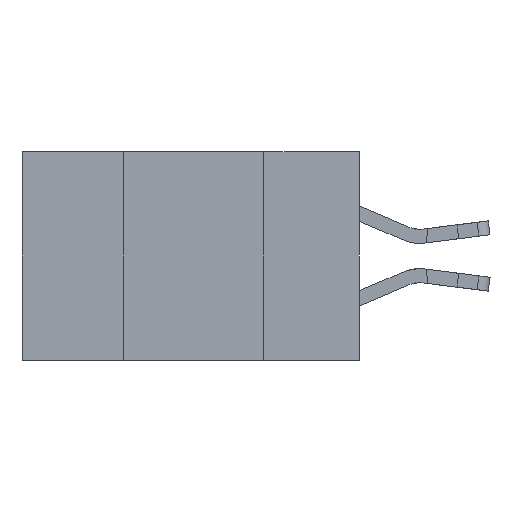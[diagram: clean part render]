
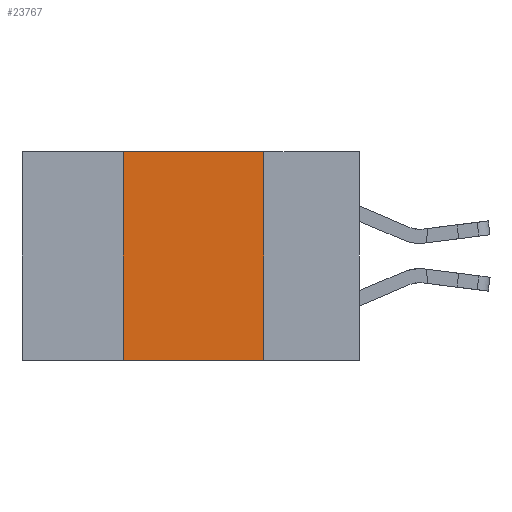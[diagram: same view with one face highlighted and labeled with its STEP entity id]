
A CAD part, left-side view. The second image highlights one B-rep face of the part: STEP entity #23767.
In plain terms, the highlighted planar face has unit normal (-1, 0, 0).
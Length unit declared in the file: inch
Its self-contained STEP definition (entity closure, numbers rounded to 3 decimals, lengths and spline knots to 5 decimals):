
#610 = VECTOR ( 'NONE', #31469, 39.37008 ) ;
#632 = ORIENTED_EDGE ( 'NONE', *, *, #25511, .T. ) ;
#822 = CARTESIAN_POINT ( 'NONE',  ( 0., 0.6, 0. ) ) ;
#1536 = VERTEX_POINT ( 'NONE', #4495 ) ;
#1778 = ORIENTED_EDGE ( 'NONE', *, *, #25185, .F. ) ;
#4495 = CARTESIAN_POINT ( 'NONE',  ( 0., 0.17, -0.37 ) ) ;
#5103 = CARTESIAN_POINT ( 'NONE',  ( 0., 0.42, -0.37 ) ) ;
#5523 = LINE ( 'NONE', #17414, #22919 ) ;
#7973 = CARTESIAN_POINT ( 'NONE',  ( 0., 0.42, 0. ) ) ;
#8697 = EDGE_LOOP ( 'NONE', ( #20877, #1778, #20939, #632 ) ) ;
#8886 = LINE ( 'NONE', #17590, #28201 ) ;
#9405 = VERTEX_POINT ( 'NONE', #5103 ) ;
#10940 = CARTESIAN_POINT ( 'NONE',  ( 0., 0.42, 0. ) ) ;
#10944 = EDGE_CURVE ( 'NONE', #9405, #20130, #28330, .T. ) ;
#11020 = DIRECTION ( 'NONE',  ( 0., 0., -1. ) ) ;
#12192 = CARTESIAN_POINT ( 'NONE',  ( 0., 0.17, 0. ) ) ;
#13394 = EDGE_CURVE ( 'NONE', #22826, #1536, #8886, .T. ) ;
#17414 = CARTESIAN_POINT ( 'NONE',  ( 0., 0.6, -0.37 ) ) ;
#17590 = CARTESIAN_POINT ( 'NONE',  ( 0., 0.17, 0. ) ) ;
#18548 = DIRECTION ( 'NONE',  ( 0., -1., 0. ) ) ;
#19758 = LINE ( 'NONE', #822, #21341 ) ;
#19857 = FACE_OUTER_BOUND ( 'NONE', #8697, .T. ) ;
#20130 = VERTEX_POINT ( 'NONE', #10940 ) ;
#20877 = ORIENTED_EDGE ( 'NONE', *, *, #13394, .F. ) ;
#20939 = ORIENTED_EDGE ( 'NONE', *, *, #10944, .F. ) ;
#21341 = VECTOR ( 'NONE', #18548, 39.37008 ) ;
#21919 = DIRECTION ( 'NONE',  ( 0., -1., 0. ) ) ;
#22826 = VERTEX_POINT ( 'NONE', #12192 ) ;
#22919 = VECTOR ( 'NONE', #21919, 39.37008 ) ;
#23592 = PLANE ( 'NONE',  #25201 ) ;
#23767 = ADVANCED_FACE ( 'NONE', ( #19857 ), #23592, .F. ) ;
#25185 = EDGE_CURVE ( 'NONE', #20130, #22826, #19758, .T. ) ;
#25201 = AXIS2_PLACEMENT_3D ( 'NONE', #28695, #26121, #11020 ) ;
#25511 = EDGE_CURVE ( 'NONE', #9405, #1536, #5523, .T. ) ;
#26121 = DIRECTION ( 'NONE',  ( 1., 0., 0. ) ) ;
#28201 = VECTOR ( 'NONE', #32635, 39.37008 ) ;
#28330 = LINE ( 'NONE', #7973, #610 ) ;
#28695 = CARTESIAN_POINT ( 'NONE',  ( 0., 0.6, 0. ) ) ;
#31469 = DIRECTION ( 'NONE',  ( 0., 0., 1. ) ) ;
#32635 = DIRECTION ( 'NONE',  ( 0., 0., -1. ) ) ;
